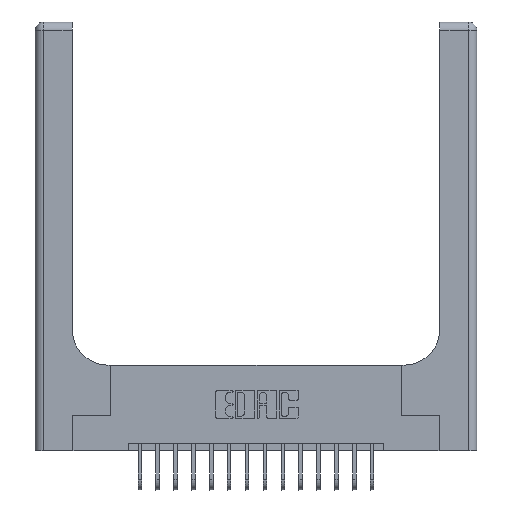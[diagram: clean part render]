
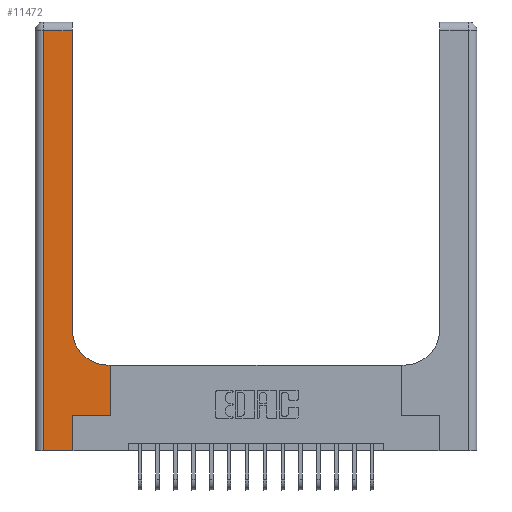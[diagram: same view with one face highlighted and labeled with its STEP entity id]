
A CAD part, top view. The second image highlights one B-rep face of the part: STEP entity #11472.
In plain terms, the highlighted planar face has unit normal (0, 0, 1).
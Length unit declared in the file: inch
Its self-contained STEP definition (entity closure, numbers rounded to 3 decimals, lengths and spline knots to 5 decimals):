
#47 = ORIENTED_EDGE ( 'NONE', *, *, #2268, .T. ) ;
#397 = CARTESIAN_POINT ( 'NONE',  ( 0.265, 0.25, 0.37 ) ) ;
#2268 = EDGE_CURVE ( 'NONE', #2909, #14546, #7605, .T. ) ;
#2398 = DIRECTION ( 'NONE',  ( 0., 1., 0. ) ) ;
#2801 = EDGE_CURVE ( 'NONE', #17626, #18029, #12206, .T. ) ;
#2909 = VERTEX_POINT ( 'NONE', #17362 ) ;
#2962 = ORIENTED_EDGE ( 'NONE', *, *, #9694, .T. ) ;
#3484 = DIRECTION ( 'NONE',  ( 0., 0., -1. ) ) ;
#3639 = CARTESIAN_POINT ( 'NONE',  ( 0.265, 0., 0.37 ) ) ;
#3761 = VECTOR ( 'NONE', #6947, 39.37008 ) ;
#4082 = CARTESIAN_POINT ( 'NONE',  ( 0.265, 0., 0.37 ) ) ;
#4314 = VECTOR ( 'NONE', #9432, 39.37008 ) ;
#4366 = CARTESIAN_POINT ( 'NONE',  ( 0.06, 0., 0.37 ) ) ;
#4696 = VECTOR ( 'NONE', #2398, 39.37008 ) ;
#4716 = FACE_OUTER_BOUND ( 'NONE', #19450, .T. ) ;
#5218 = EDGE_CURVE ( 'NONE', #16701, #17626, #13426, .T. ) ;
#5431 = DIRECTION ( 'NONE',  ( 1., 0., 0. ) ) ;
#5516 = LINE ( 'NONE', #11589, #3761 ) ;
#5734 = CARTESIAN_POINT ( 'NONE',  ( 0.26, 0.6, 0.37 ) ) ;
#6246 = CARTESIAN_POINT ( 'NONE',  ( 0.265, 0.25, 0.37 ) ) ;
#6947 = DIRECTION ( 'NONE',  ( 0., 1., 0. ) ) ;
#7605 = LINE ( 'NONE', #10802, #11593 ) ;
#7624 = ORIENTED_EDGE ( 'NONE', *, *, #18273, .T. ) ;
#8118 = VERTEX_POINT ( 'NONE', #19839 ) ;
#9082 = VECTOR ( 'NONE', #17591, 39.37008 ) ;
#9432 = DIRECTION ( 'NONE',  ( 1., 0., 0. ) ) ;
#9694 = EDGE_CURVE ( 'NONE', #14331, #8118, #19515, .T. ) ;
#9702 = EDGE_CURVE ( 'NONE', #8118, #16085, #13614, .T. ) ;
#10369 = CARTESIAN_POINT ( 'NONE',  ( 0.51, 0.85, 0.37 ) ) ;
#10472 = ORIENTED_EDGE ( 'NONE', *, *, #2801, .T. ) ;
#10702 = AXIS2_PLACEMENT_3D ( 'NONE', #14497, #3484, #14099 ) ;
#10802 = CARTESIAN_POINT ( 'NONE',  ( 0.06, 3., 0.37 ) ) ;
#10938 = ORIENTED_EDGE ( 'NONE', *, *, #9702, .T. ) ;
#11003 = CARTESIAN_POINT ( 'NONE',  ( 0.26, 2.94, 0.37 ) ) ;
#11315 = PLANE ( 'NONE',  #10702 ) ;
#11317 = LINE ( 'NONE', #15735, #9082 ) ;
#11472 = ADVANCED_FACE ( 'NONE', ( #4716 ), #11315, .F. ) ;
#11589 = CARTESIAN_POINT ( 'NONE',  ( 0.528, 0.25, 0.37 ) ) ;
#11593 = VECTOR ( 'NONE', #12446, 39.37008 ) ;
#11909 = DIRECTION ( 'NONE',  ( 0., 1., 0. ) ) ;
#11944 = ORIENTED_EDGE ( 'NONE', *, *, #12725, .T. ) ;
#11969 = LINE ( 'NONE', #18044, #18614 ) ;
#12017 = DIRECTION ( 'NONE',  ( -1., 0., 0. ) ) ;
#12206 = LINE ( 'NONE', #6246, #4314 ) ;
#12446 = DIRECTION ( 'NONE',  ( 0., -1., 0. ) ) ;
#12492 = EDGE_CURVE ( 'NONE', #17602, #2909, #11969, .T. ) ;
#12621 = VECTOR ( 'NONE', #12017, 39.37008 ) ;
#12725 = EDGE_CURVE ( 'NONE', #14546, #16701, #11317, .T. ) ;
#13253 = VECTOR ( 'NONE', #11909, 39.37008 ) ;
#13426 = LINE ( 'NONE', #3639, #4696 ) ;
#13614 = CIRCLE ( 'NONE', #18218, 0.25 ) ;
#14099 = DIRECTION ( 'NONE',  ( -1., 0., 0. ) ) ;
#14331 = VERTEX_POINT ( 'NONE', #14501 ) ;
#14497 = CARTESIAN_POINT ( 'NONE',  ( 0., 3., 0.37 ) ) ;
#14501 = CARTESIAN_POINT ( 'NONE',  ( 0.528, 0.6, 0.37 ) ) ;
#14546 = VERTEX_POINT ( 'NONE', #4366 ) ;
#15403 = CARTESIAN_POINT ( 'NONE',  ( 0.528, 0.25, 0.37 ) ) ;
#15735 = CARTESIAN_POINT ( 'NONE',  ( 0., 0., 0.37 ) ) ;
#16085 = VERTEX_POINT ( 'NONE', #18108 ) ;
#16685 = ORIENTED_EDGE ( 'NONE', *, *, #16688, .T. ) ;
#16688 = EDGE_CURVE ( 'NONE', #16085, #17602, #16740, .T. ) ;
#16701 = VERTEX_POINT ( 'NONE', #4082 ) ;
#16740 = LINE ( 'NONE', #19718, #13253 ) ;
#17127 = ORIENTED_EDGE ( 'NONE', *, *, #5218, .T. ) ;
#17362 = CARTESIAN_POINT ( 'NONE',  ( 0.06, 2.94, 0.37 ) ) ;
#17591 = DIRECTION ( 'NONE',  ( 1., 0., 0. ) ) ;
#17602 = VERTEX_POINT ( 'NONE', #11003 ) ;
#17626 = VERTEX_POINT ( 'NONE', #397 ) ;
#18029 = VERTEX_POINT ( 'NONE', #15403 ) ;
#18044 = CARTESIAN_POINT ( 'NONE',  ( 0., 2.94, 0.37 ) ) ;
#18108 = CARTESIAN_POINT ( 'NONE',  ( 0.26, 0.85, 0.37 ) ) ;
#18218 = AXIS2_PLACEMENT_3D ( 'NONE', #10369, #19919, #5431 ) ;
#18273 = EDGE_CURVE ( 'NONE', #18029, #14331, #5516, .T. ) ;
#18301 = ORIENTED_EDGE ( 'NONE', *, *, #12492, .T. ) ;
#18614 = VECTOR ( 'NONE', #20259, 39.37008 ) ;
#19450 = EDGE_LOOP ( 'NONE', ( #16685, #18301, #47, #11944, #17127, #10472, #7624, #2962, #10938 ) ) ;
#19515 = LINE ( 'NONE', #5734, #12621 ) ;
#19718 = CARTESIAN_POINT ( 'NONE',  ( 0.26, 3., 0.37 ) ) ;
#19839 = CARTESIAN_POINT ( 'NONE',  ( 0.51, 0.6, 0.37 ) ) ;
#19919 = DIRECTION ( 'NONE',  ( 0., 0., -1. ) ) ;
#20259 = DIRECTION ( 'NONE',  ( -1., 0., 0. ) ) ;
